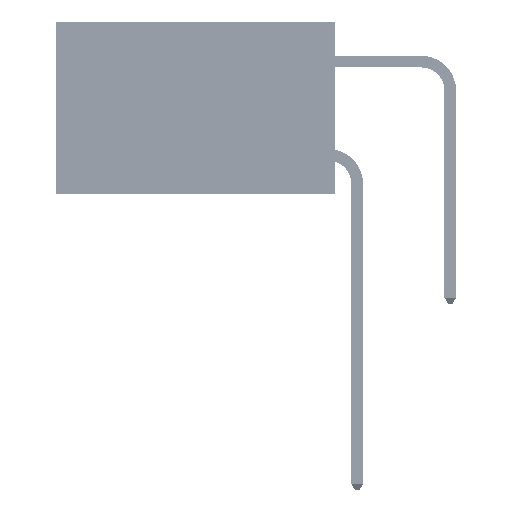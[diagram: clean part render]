
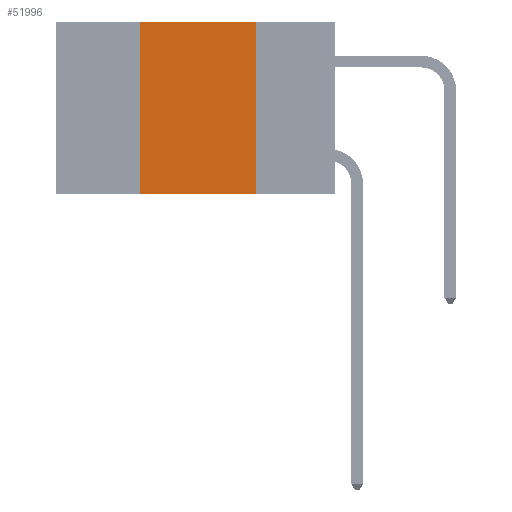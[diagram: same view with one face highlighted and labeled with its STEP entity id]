
A CAD part, left-side view. The second image highlights one B-rep face of the part: STEP entity #51996.
In plain terms, the highlighted planar face has unit normal (-1, 0, 0).
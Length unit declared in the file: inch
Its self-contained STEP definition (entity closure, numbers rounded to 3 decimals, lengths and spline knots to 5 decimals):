
#417 = VERTEX_POINT ( 'NONE', #30119 ) ;
#3273 = ORIENTED_EDGE ( 'NONE', *, *, #53359, .F. ) ;
#4429 = VECTOR ( 'NONE', #16131, 39.37008 ) ;
#4496 = ORIENTED_EDGE ( 'NONE', *, *, #6434, .T. ) ;
#5312 = AXIS2_PLACEMENT_3D ( 'NONE', #18851, #35320, #51818 ) ;
#6434 = EDGE_CURVE ( 'NONE', #34074, #26496, #24349, .T. ) ;
#8089 = CARTESIAN_POINT ( 'NONE',  ( 0., 0.42, 0. ) ) ;
#11807 = CARTESIAN_POINT ( 'NONE',  ( 0., 0.6, 0. ) ) ;
#16131 = DIRECTION ( 'NONE',  ( 0., -1., 0. ) ) ;
#16252 = CARTESIAN_POINT ( 'NONE',  ( 0., 0.6, -0.37 ) ) ;
#18851 = CARTESIAN_POINT ( 'NONE',  ( 0., 0.6, 0. ) ) ;
#20637 = ORIENTED_EDGE ( 'NONE', *, *, #39792, .F. ) ;
#20648 = VECTOR ( 'NONE', #45740, 39.37008 ) ;
#23810 = DIRECTION ( 'NONE',  ( 0., 0., 1. ) ) ;
#23829 = DIRECTION ( 'NONE',  ( 0., -1., 0. ) ) ;
#24349 = LINE ( 'NONE', #16252, #44168 ) ;
#25668 = CARTESIAN_POINT ( 'NONE',  ( 0., 0.17, -0.37 ) ) ;
#26316 = EDGE_CURVE ( 'NONE', #34074, #33540, #28416, .T. ) ;
#26496 = VERTEX_POINT ( 'NONE', #25668 ) ;
#26958 = FACE_OUTER_BOUND ( 'NONE', #41948, .T. ) ;
#28416 = LINE ( 'NONE', #8089, #51156 ) ;
#29105 = ORIENTED_EDGE ( 'NONE', *, *, #26316, .F. ) ;
#29755 = CARTESIAN_POINT ( 'NONE',  ( 0., 0.42, 0. ) ) ;
#30119 = CARTESIAN_POINT ( 'NONE',  ( 0., 0.17, 0. ) ) ;
#33540 = VERTEX_POINT ( 'NONE', #29755 ) ;
#34074 = VERTEX_POINT ( 'NONE', #42925 ) ;
#35320 = DIRECTION ( 'NONE',  ( 1., 0., 0. ) ) ;
#36392 = LINE ( 'NONE', #11807, #4429 ) ;
#37358 = CARTESIAN_POINT ( 'NONE',  ( 0., 0.17, 0. ) ) ;
#39792 = EDGE_CURVE ( 'NONE', #417, #26496, #48734, .T. ) ;
#41948 = EDGE_LOOP ( 'NONE', ( #20637, #3273, #29105, #4496 ) ) ;
#42925 = CARTESIAN_POINT ( 'NONE',  ( 0., 0.42, -0.37 ) ) ;
#43439 = PLANE ( 'NONE',  #5312 ) ;
#44168 = VECTOR ( 'NONE', #23829, 39.37008 ) ;
#45740 = DIRECTION ( 'NONE',  ( 0., 0., -1. ) ) ;
#48734 = LINE ( 'NONE', #37358, #20648 ) ;
#51156 = VECTOR ( 'NONE', #23810, 39.37008 ) ;
#51818 = DIRECTION ( 'NONE',  ( 0., 0., -1. ) ) ;
#51996 = ADVANCED_FACE ( 'NONE', ( #26958 ), #43439, .F. ) ;
#53359 = EDGE_CURVE ( 'NONE', #33540, #417, #36392, .T. ) ;
